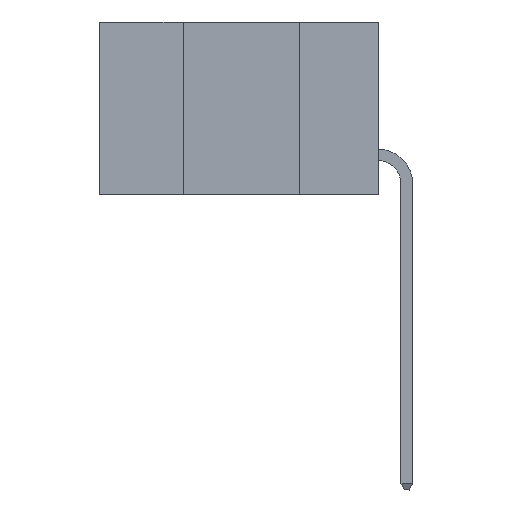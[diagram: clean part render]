
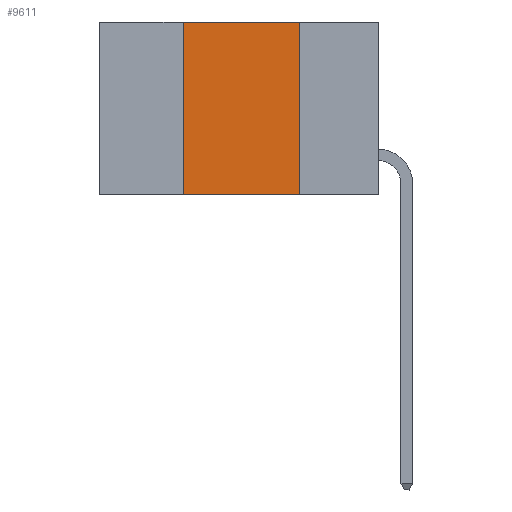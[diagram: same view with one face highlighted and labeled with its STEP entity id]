
A CAD part, left-side view. The second image highlights one B-rep face of the part: STEP entity #9611.
In plain terms, the highlighted planar face has unit normal (-1, 0, 0).
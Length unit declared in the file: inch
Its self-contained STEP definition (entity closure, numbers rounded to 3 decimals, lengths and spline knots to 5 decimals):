
#315 = CARTESIAN_POINT ( 'NONE',  ( 0., 0.6, -0.37 ) ) ;
#888 = CARTESIAN_POINT ( 'NONE',  ( 0., 0.6, 0. ) ) ;
#924 = VECTOR ( 'NONE', #12434, 39.37008 ) ;
#1716 = VERTEX_POINT ( 'NONE', #9514 ) ;
#2026 = LINE ( 'NONE', #16102, #8824 ) ;
#2182 = DIRECTION ( 'NONE',  ( 1., 0., 0. ) ) ;
#2345 = CARTESIAN_POINT ( 'NONE',  ( 0., 0.42, -0.37 ) ) ;
#3688 = AXIS2_PLACEMENT_3D ( 'NONE', #888, #2182, #11155 ) ;
#3941 = EDGE_CURVE ( 'NONE', #5882, #5867, #2026, .T. ) ;
#4803 = DIRECTION ( 'NONE',  ( 0., 0., -1. ) ) ;
#5269 = VERTEX_POINT ( 'NONE', #2345 ) ;
#5849 = CARTESIAN_POINT ( 'NONE',  ( 0., 0.17, 0. ) ) ;
#5867 = VERTEX_POINT ( 'NONE', #5849 ) ;
#5882 = VERTEX_POINT ( 'NONE', #12715 ) ;
#5945 = LINE ( 'NONE', #315, #15825 ) ;
#6348 = LINE ( 'NONE', #8579, #9364 ) ;
#6356 = ORIENTED_EDGE ( 'NONE', *, *, #15850, .F. ) ;
#6896 = EDGE_CURVE ( 'NONE', #5867, #1716, #6348, .T. ) ;
#8150 = ORIENTED_EDGE ( 'NONE', *, *, #3941, .F. ) ;
#8557 = PLANE ( 'NONE',  #3688 ) ;
#8579 = CARTESIAN_POINT ( 'NONE',  ( 0., 0.17, 0. ) ) ;
#8596 = ORIENTED_EDGE ( 'NONE', *, *, #16184, .T. ) ;
#8655 = ORIENTED_EDGE ( 'NONE', *, *, #6896, .F. ) ;
#8824 = VECTOR ( 'NONE', #16170, 39.37008 ) ;
#9364 = VECTOR ( 'NONE', #4803, 39.37008 ) ;
#9514 = CARTESIAN_POINT ( 'NONE',  ( 0., 0.17, -0.37 ) ) ;
#9611 = ADVANCED_FACE ( 'NONE', ( #15163 ), #8557, .F. ) ;
#10620 = DIRECTION ( 'NONE',  ( 0., -1., 0. ) ) ;
#11147 = CARTESIAN_POINT ( 'NONE',  ( 0., 0.42, 0. ) ) ;
#11155 = DIRECTION ( 'NONE',  ( 0., 0., -1. ) ) ;
#12117 = EDGE_LOOP ( 'NONE', ( #8655, #8150, #6356, #8596 ) ) ;
#12434 = DIRECTION ( 'NONE',  ( 0., 0., 1. ) ) ;
#12715 = CARTESIAN_POINT ( 'NONE',  ( 0., 0.42, 0. ) ) ;
#14634 = LINE ( 'NONE', #11147, #924 ) ;
#15163 = FACE_OUTER_BOUND ( 'NONE', #12117, .T. ) ;
#15825 = VECTOR ( 'NONE', #10620, 39.37008 ) ;
#15850 = EDGE_CURVE ( 'NONE', #5269, #5882, #14634, .T. ) ;
#16102 = CARTESIAN_POINT ( 'NONE',  ( 0., 0.6, 0. ) ) ;
#16170 = DIRECTION ( 'NONE',  ( 0., -1., 0. ) ) ;
#16184 = EDGE_CURVE ( 'NONE', #5269, #1716, #5945, .T. ) ;
